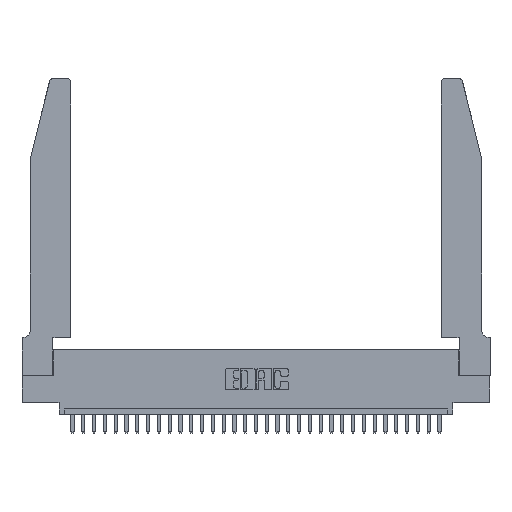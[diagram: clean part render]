
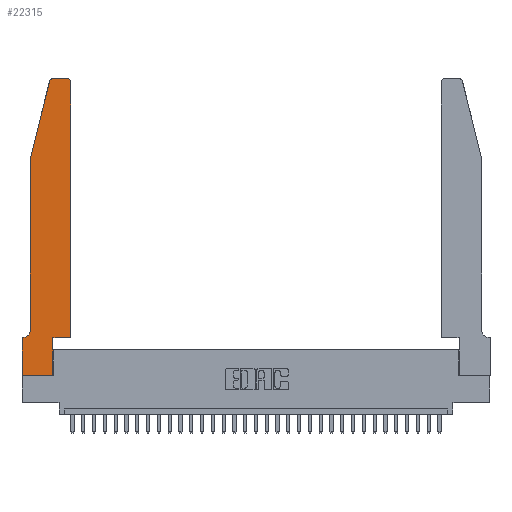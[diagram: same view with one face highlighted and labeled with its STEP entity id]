
A CAD part, top view. The second image highlights one B-rep face of the part: STEP entity #22315.
In plain terms, the highlighted planar face has unit normal (0, 0, 1).
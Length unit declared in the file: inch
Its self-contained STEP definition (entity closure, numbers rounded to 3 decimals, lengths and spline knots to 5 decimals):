
#9 = DIRECTION ( 'NONE',  ( 0., 0., 1. ) ) ;
#78 = EDGE_CURVE ( 'NONE', #27266, #4559, #8013, .T. ) ;
#222 = CIRCLE ( 'NONE', #10933, 0.03 ) ;
#479 = CARTESIAN_POINT ( 'NONE',  ( 0., 0.35, 0.37 ) ) ;
#701 = PLANE ( 'NONE',  #31828 ) ;
#990 = CARTESIAN_POINT ( 'NONE',  ( 0.2605, 2.75, 0.37 ) ) ;
#1095 = DIRECTION ( 'NONE',  ( -0.239, -0.971, 0. ) ) ;
#1160 = CARTESIAN_POINT ( 'NONE',  ( 0., 0., 0.37 ) ) ;
#1289 = CIRCLE ( 'NONE', #20524, 0.07 ) ;
#2301 = CARTESIAN_POINT ( 'NONE',  ( 0.2865, 0.35, 0.37 ) ) ;
#2348 = CARTESIAN_POINT ( 'NONE',  ( 0.0055, 0.35, 0.37 ) ) ;
#2762 = VECTOR ( 'NONE', #11997, 39.37008 ) ;
#2811 = VERTEX_POINT ( 'NONE', #31463 ) ;
#2914 = VECTOR ( 'NONE', #26534, 39.37008 ) ;
#4077 = VECTOR ( 'NONE', #30577, 39.37008 ) ;
#4376 = VECTOR ( 'NONE', #23487, 39.37008 ) ;
#4559 = VERTEX_POINT ( 'NONE', #14347 ) ;
#5113 = LINE ( 'NONE', #16002, #2762 ) ;
#5257 = DIRECTION ( 'NONE',  ( 0., 1., 0. ) ) ;
#5367 = CARTESIAN_POINT ( 'NONE',  ( 0.284, 2.72, 0.37 ) ) ;
#5745 = LINE ( 'NONE', #30982, #11686 ) ;
#5950 = LINE ( 'NONE', #30521, #4376 ) ;
#6115 = EDGE_CURVE ( 'NONE', #29682, #28338, #30476, .T. ) ;
#6165 = DIRECTION ( 'NONE',  ( 0., 1., 0. ) ) ;
#6629 = DIRECTION ( 'NONE',  ( 1., 0., 0. ) ) ;
#7023 = DIRECTION ( 'NONE',  ( 0., -1., 0. ) ) ;
#7057 = VECTOR ( 'NONE', #5257, 39.37008 ) ;
#7703 = EDGE_CURVE ( 'NONE', #12394, #2811, #222, .T. ) ;
#8013 = LINE ( 'NONE', #1160, #2914 ) ;
#8128 = DIRECTION ( 'NONE',  ( 1., 0., 0. ) ) ;
#8460 = EDGE_LOOP ( 'NONE', ( #24890, #23521, #11707, #12270, #11546, #8468, #8880, #16066, #31727, #27373, #16182, #22854 ) ) ;
#8468 = ORIENTED_EDGE ( 'NONE', *, *, #19640, .T. ) ;
#8880 = ORIENTED_EDGE ( 'NONE', *, *, #78, .T. ) ;
#9422 = EDGE_CURVE ( 'NONE', #28338, #15624, #1289, .T. ) ;
#9475 = EDGE_CURVE ( 'NONE', #4559, #19243, #5950, .T. ) ;
#10302 = EDGE_CURVE ( 'NONE', #19243, #20018, #11409, .T. ) ;
#10605 = CIRCLE ( 'NONE', #14015, 0.03 ) ;
#10933 = AXIS2_PLACEMENT_3D ( 'NONE', #32256, #9, #17472 ) ;
#11207 = LINE ( 'NONE', #990, #4077 ) ;
#11409 = LINE ( 'NONE', #29802, #7057 ) ;
#11546 = ORIENTED_EDGE ( 'NONE', *, *, #9422, .T. ) ;
#11686 = VECTOR ( 'NONE', #6165, 39.37008 ) ;
#11707 = ORIENTED_EDGE ( 'NONE', *, *, #31134, .T. ) ;
#11997 = DIRECTION ( 'NONE',  ( -1., 0., 0. ) ) ;
#12270 = ORIENTED_EDGE ( 'NONE', *, *, #6115, .T. ) ;
#12394 = VERTEX_POINT ( 'NONE', #16244 ) ;
#12503 = LINE ( 'NONE', #13685, #27990 ) ;
#12942 = LINE ( 'NONE', #21665, #19158 ) ;
#13532 = CARTESIAN_POINT ( 'NONE',  ( 0.0055, 0.42, 0.37 ) ) ;
#13685 = CARTESIAN_POINT ( 'NONE',  ( 0.0755, 2., 0.37 ) ) ;
#14015 = AXIS2_PLACEMENT_3D ( 'NONE', #5367, #15680, #8128 ) ;
#14208 = CARTESIAN_POINT ( 'NONE',  ( 0.0755, 2., 0.37 ) ) ;
#14302 = VERTEX_POINT ( 'NONE', #26792 ) ;
#14347 = CARTESIAN_POINT ( 'NONE',  ( 0., 0., 0.37 ) ) ;
#15624 = VERTEX_POINT ( 'NONE', #2348 ) ;
#15680 = DIRECTION ( 'NONE',  ( 0., 0., 1. ) ) ;
#16002 = CARTESIAN_POINT ( 'NONE',  ( 0.0755, 0.35, 0.37 ) ) ;
#16066 = ORIENTED_EDGE ( 'NONE', *, *, #9475, .T. ) ;
#16182 = ORIENTED_EDGE ( 'NONE', *, *, #19444, .T. ) ;
#16244 = CARTESIAN_POINT ( 'NONE',  ( 0.4505, 2.72, 0.37 ) ) ;
#17472 = DIRECTION ( 'NONE',  ( 1., 0., 0. ) ) ;
#18105 = CARTESIAN_POINT ( 'NONE',  ( 0.2865, 0., 0.37 ) ) ;
#19158 = VECTOR ( 'NONE', #6629, 39.37008 ) ;
#19243 = VERTEX_POINT ( 'NONE', #18105 ) ;
#19444 = EDGE_CURVE ( 'NONE', #14302, #12394, #5745, .T. ) ;
#19640 = EDGE_CURVE ( 'NONE', #15624, #27266, #5113, .T. ) ;
#19688 = VERTEX_POINT ( 'NONE', #22544 ) ;
#20018 = VERTEX_POINT ( 'NONE', #2301 ) ;
#20262 = CARTESIAN_POINT ( 'NONE',  ( 0.25487, 2.72718, 0.37 ) ) ;
#20524 = AXIS2_PLACEMENT_3D ( 'NONE', #13532, #20840, #20742 ) ;
#20742 = DIRECTION ( 'NONE',  ( -1., 0., 0. ) ) ;
#20840 = DIRECTION ( 'NONE',  ( 0., 0., -1. ) ) ;
#21665 = CARTESIAN_POINT ( 'NONE',  ( 0.4505, 0.35, 0.37 ) ) ;
#22315 = ADVANCED_FACE ( 'NONE', ( #30247 ), #701, .T. ) ;
#22544 = CARTESIAN_POINT ( 'NONE',  ( 0.284, 2.75, 0.37 ) ) ;
#22854 = ORIENTED_EDGE ( 'NONE', *, *, #7703, .T. ) ;
#22971 = EDGE_CURVE ( 'NONE', #2811, #19688, #11207, .T. ) ;
#23487 = DIRECTION ( 'NONE',  ( 1., 0., 0. ) ) ;
#23521 = ORIENTED_EDGE ( 'NONE', *, *, #25338, .T. ) ;
#23563 = CARTESIAN_POINT ( 'NONE',  ( 0.0755, 0.42, 0.37 ) ) ;
#24890 = ORIENTED_EDGE ( 'NONE', *, *, #22971, .T. ) ;
#25338 = EDGE_CURVE ( 'NONE', #19688, #27211, #10605, .T. ) ;
#26534 = DIRECTION ( 'NONE',  ( 0., -1., 0. ) ) ;
#26792 = CARTESIAN_POINT ( 'NONE',  ( 0.4505, 0.35, 0.37 ) ) ;
#27211 = VERTEX_POINT ( 'NONE', #20262 ) ;
#27266 = VERTEX_POINT ( 'NONE', #27905 ) ;
#27373 = ORIENTED_EDGE ( 'NONE', *, *, #29026, .T. ) ;
#27390 = VECTOR ( 'NONE', #7023, 39.37008 ) ;
#27824 = DIRECTION ( 'NONE',  ( 0., 0., 1. ) ) ;
#27905 = CARTESIAN_POINT ( 'NONE',  ( 0., 0.35, 0.37 ) ) ;
#27990 = VECTOR ( 'NONE', #1095, 39.37008 ) ;
#28338 = VERTEX_POINT ( 'NONE', #23563 ) ;
#28906 = CARTESIAN_POINT ( 'NONE',  ( 0.0755, 2., 0.37 ) ) ;
#29026 = EDGE_CURVE ( 'NONE', #20018, #14302, #12942, .T. ) ;
#29682 = VERTEX_POINT ( 'NONE', #14208 ) ;
#29802 = CARTESIAN_POINT ( 'NONE',  ( 0.2865, 0.35, 0.37 ) ) ;
#30247 = FACE_OUTER_BOUND ( 'NONE', #8460, .T. ) ;
#30404 = DIRECTION ( 'NONE',  ( 1., 0., 0. ) ) ;
#30476 = LINE ( 'NONE', #28906, #27390 ) ;
#30521 = CARTESIAN_POINT ( 'NONE',  ( 0., 0., 0.37 ) ) ;
#30577 = DIRECTION ( 'NONE',  ( -1., 0., 0. ) ) ;
#30982 = CARTESIAN_POINT ( 'NONE',  ( 0.4505, 0.35, 0.37 ) ) ;
#31134 = EDGE_CURVE ( 'NONE', #27211, #29682, #12503, .T. ) ;
#31463 = CARTESIAN_POINT ( 'NONE',  ( 0.4205, 2.75, 0.37 ) ) ;
#31727 = ORIENTED_EDGE ( 'NONE', *, *, #10302, .T. ) ;
#31828 = AXIS2_PLACEMENT_3D ( 'NONE', #479, #27824, #30404 ) ;
#32256 = CARTESIAN_POINT ( 'NONE',  ( 0.4205, 2.72, 0.37 ) ) ;
